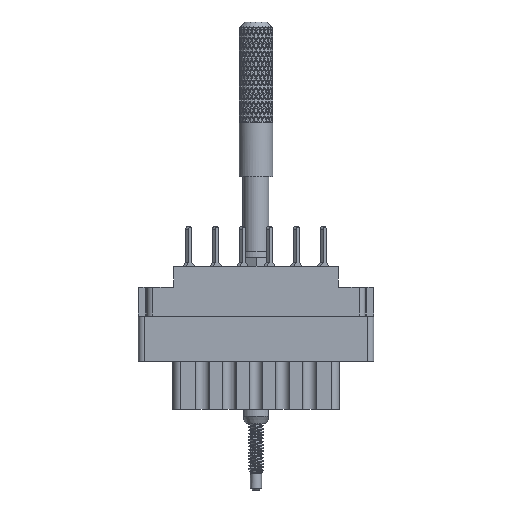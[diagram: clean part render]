
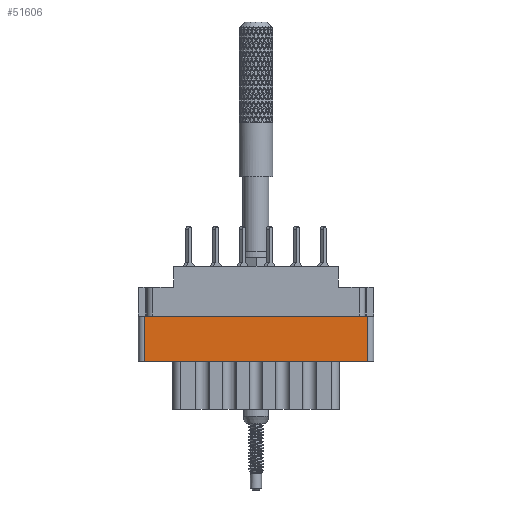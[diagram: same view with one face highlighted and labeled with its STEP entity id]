
A CAD part, front view. The second image highlights one B-rep face of the part: STEP entity #51606.
In plain terms, the highlighted planar face has unit normal (0, -1, 0).
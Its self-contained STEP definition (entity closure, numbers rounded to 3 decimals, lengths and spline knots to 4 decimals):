
#2243 = DIRECTION ( 'NONE',  ( 0., 0., 1. ) ) ;
#4059 = CARTESIAN_POINT ( 'NONE',  ( 0.624, -0.343, -0.798 ) ) ;
#4493 = CARTESIAN_POINT ( 'NONE',  ( -0.624, -0.343, -0.798 ) ) ;
#5887 = LINE ( 'NONE', #4059, #103265 ) ;
#6663 = CARTESIAN_POINT ( 'NONE',  ( 0.624, -0.343, -0.277 ) ) ;
#18384 = FACE_OUTER_BOUND ( 'NONE', #136375, .T. ) ;
#19250 = VERTEX_POINT ( 'NONE', #6663 ) ;
#19705 = AXIS2_PLACEMENT_3D ( 'NONE', #4493, #42506, #173083 ) ;
#21903 = CARTESIAN_POINT ( 'NONE',  ( -0.624, -0.343, -0.798 ) ) ;
#25732 = ORIENTED_EDGE ( 'NONE', *, *, #166706, .F. ) ;
#28763 = DIRECTION ( 'NONE',  ( -1., 0., 0. ) ) ;
#34657 = CARTESIAN_POINT ( 'NONE',  ( -0.624, -0.343, -0.277 ) ) ;
#36690 = DIRECTION ( 'NONE',  ( 0., 0., 1. ) ) ;
#37019 = EDGE_CURVE ( 'NONE', #168565, #129325, #41735, .T. ) ;
#41735 = LINE ( 'NONE', #82496, #126492 ) ;
#42506 = DIRECTION ( 'NONE',  ( 0., -1., 0. ) ) ;
#46263 = VERTEX_POINT ( 'NONE', #34657 ) ;
#51606 = ADVANCED_FACE ( 'NONE', ( #18384 ), #131355, .T. ) ;
#66347 = EDGE_CURVE ( 'NONE', #168565, #19250, #5887, .T. ) ;
#76229 = ORIENTED_EDGE ( 'NONE', *, *, #86634, .F. ) ;
#79331 = CARTESIAN_POINT ( 'NONE',  ( 0.624, -0.343, -0.529 ) ) ;
#82496 = CARTESIAN_POINT ( 'NONE',  ( 0.624, -0.343, -0.529 ) ) ;
#86634 = EDGE_CURVE ( 'NONE', #46263, #19250, #145450, .T. ) ;
#87087 = DIRECTION ( 'NONE',  ( 1., 0., 0. ) ) ;
#90639 = CARTESIAN_POINT ( 'NONE',  ( -0.624, -0.343, -0.529 ) ) ;
#93146 = LINE ( 'NONE', #21903, #112621 ) ;
#95361 = VECTOR ( 'NONE', #87087, 39.3701 ) ;
#103265 = VECTOR ( 'NONE', #2243, 39.3701 ) ;
#112621 = VECTOR ( 'NONE', #36690, 39.3701 ) ;
#125746 = ORIENTED_EDGE ( 'NONE', *, *, #66347, .T. ) ;
#126492 = VECTOR ( 'NONE', #28763, 39.3701 ) ;
#129325 = VERTEX_POINT ( 'NONE', #90639 ) ;
#131355 = PLANE ( 'NONE',  #19705 ) ;
#136375 = EDGE_LOOP ( 'NONE', ( #25732, #142597, #125746, #76229 ) ) ;
#142597 = ORIENTED_EDGE ( 'NONE', *, *, #37019, .F. ) ;
#145450 = LINE ( 'NONE', #171440, #95361 ) ;
#166706 = EDGE_CURVE ( 'NONE', #129325, #46263, #93146, .T. ) ;
#168565 = VERTEX_POINT ( 'NONE', #79331 ) ;
#171440 = CARTESIAN_POINT ( 'NONE',  ( -0.656, -0.343, -0.277 ) ) ;
#173083 = DIRECTION ( 'NONE',  ( 0., 0., -1. ) ) ;
